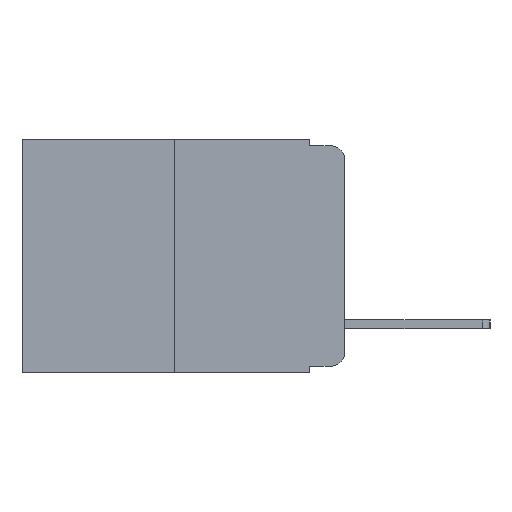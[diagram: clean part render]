
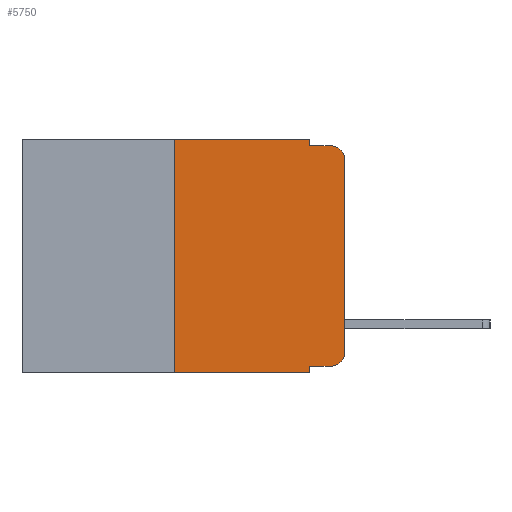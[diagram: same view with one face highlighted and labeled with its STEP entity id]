
A CAD part, left-side view. The second image highlights one B-rep face of the part: STEP entity #5750.
In plain terms, the highlighted planar face has unit normal (-1, 0, 0).
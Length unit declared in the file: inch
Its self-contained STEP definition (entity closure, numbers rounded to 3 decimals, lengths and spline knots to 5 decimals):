
#262 = DIRECTION ( 'NONE',  ( 0., -1., 0. ) ) ;
#375 = ORIENTED_EDGE ( 'NONE', *, *, #10968, .F. ) ;
#394 = ORIENTED_EDGE ( 'NONE', *, *, #12200, .T. ) ;
#423 = ORIENTED_EDGE ( 'NONE', *, *, #14077, .T. ) ;
#573 = DIRECTION ( 'NONE',  ( 0., 0., 1. ) ) ;
#577 = ORIENTED_EDGE ( 'NONE', *, *, #7756, .F. ) ;
#736 = LINE ( 'NONE', #17203, #4063 ) ;
#753 = VECTOR ( 'NONE', #2154, 39.37008 ) ;
#880 = FACE_OUTER_BOUND ( 'NONE', #13927, .T. ) ;
#1391 = CIRCLE ( 'NONE', #11927, 0.02 ) ;
#1457 = VECTOR ( 'NONE', #6926, 39.37008 ) ;
#1819 = EDGE_CURVE ( 'NONE', #5526, #11667, #8682, .T. ) ;
#2154 = DIRECTION ( 'NONE',  ( 0., -1., 0. ) ) ;
#2223 = DIRECTION ( 'NONE',  ( -1., 0., 0. ) ) ;
#2265 = CARTESIAN_POINT ( 'NONE',  ( 0., 0.051, -0.01 ) ) ;
#2388 = EDGE_CURVE ( 'NONE', #11225, #7381, #5765, .T. ) ;
#2497 = CARTESIAN_POINT ( 'NONE',  ( 0., 0.051, 0. ) ) ;
#2544 = ORIENTED_EDGE ( 'NONE', *, *, #2853, .T. ) ;
#2697 = DIRECTION ( 'NONE',  ( 1., 0., 0. ) ) ;
#2853 = EDGE_CURVE ( 'NONE', #13349, #5893, #15916, .T. ) ;
#2949 = CARTESIAN_POINT ( 'NONE',  ( 0., 0., -0.03 ) ) ;
#3145 = CARTESIAN_POINT ( 'NONE',  ( 0., 0.25, 0. ) ) ;
#3374 = VECTOR ( 'NONE', #5452, 39.37008 ) ;
#3471 = ORIENTED_EDGE ( 'NONE', *, *, #8211, .F. ) ;
#3778 = CARTESIAN_POINT ( 'NONE',  ( 0., 0.02, -0.03 ) ) ;
#4063 = VECTOR ( 'NONE', #573, 39.37008 ) ;
#4452 = EDGE_CURVE ( 'NONE', #11667, #6717, #1391, .T. ) ;
#4487 = CARTESIAN_POINT ( 'NONE',  ( 0., 0.051, -0.343 ) ) ;
#4535 = DIRECTION ( 'NONE',  ( -1., 0., 0. ) ) ;
#4559 = DIRECTION ( 'NONE',  ( 0., 0., -1. ) ) ;
#4885 = VECTOR ( 'NONE', #6963, 39.37008 ) ;
#4895 = VECTOR ( 'NONE', #16625, 39.37008 ) ;
#5059 = ORIENTED_EDGE ( 'NONE', *, *, #4452, .T. ) ;
#5452 = DIRECTION ( 'NONE',  ( 0., 0., -1. ) ) ;
#5526 = VERTEX_POINT ( 'NONE', #15768 ) ;
#5626 = CARTESIAN_POINT ( 'NONE',  ( 0., 0.02, -0.333 ) ) ;
#5638 = VECTOR ( 'NONE', #262, 39.37008 ) ;
#5750 = ADVANCED_FACE ( 'NONE', ( #880 ), #16596, .F. ) ;
#5765 = LINE ( 'NONE', #11553, #1457 ) ;
#5893 = VERTEX_POINT ( 'NONE', #4487 ) ;
#6717 = VERTEX_POINT ( 'NONE', #7292 ) ;
#6846 = CIRCLE ( 'NONE', #14888, 0.02 ) ;
#6926 = DIRECTION ( 'NONE',  ( 0., 0., -1. ) ) ;
#6963 = DIRECTION ( 'NONE',  ( 0., 0., 1. ) ) ;
#7292 = CARTESIAN_POINT ( 'NONE',  ( 0., 0.02, -0.01 ) ) ;
#7381 = VERTEX_POINT ( 'NONE', #2265 ) ;
#7756 = EDGE_CURVE ( 'NONE', #7381, #6717, #13536, .T. ) ;
#7896 = CARTESIAN_POINT ( 'NONE',  ( 0., 0., 0. ) ) ;
#7938 = LINE ( 'NONE', #10737, #753 ) ;
#7962 = ORIENTED_EDGE ( 'NONE', *, *, #1819, .T. ) ;
#8211 = EDGE_CURVE ( 'NONE', #11590, #5893, #14610, .T. ) ;
#8437 = VERTEX_POINT ( 'NONE', #3145 ) ;
#8682 = LINE ( 'NONE', #7896, #4885 ) ;
#9321 = ORIENTED_EDGE ( 'NONE', *, *, #11308, .F. ) ;
#10296 = CARTESIAN_POINT ( 'NONE',  ( 0., 0.051, 0. ) ) ;
#10561 = AXIS2_PLACEMENT_3D ( 'NONE', #11285, #2697, #12663 ) ;
#10737 = CARTESIAN_POINT ( 'NONE',  ( 0., 0.473, 0. ) ) ;
#10819 = CARTESIAN_POINT ( 'NONE',  ( 0., 0.02, -0.313 ) ) ;
#10968 = EDGE_CURVE ( 'NONE', #8437, #11225, #7938, .T. ) ;
#11091 = CARTESIAN_POINT ( 'NONE',  ( 0., 0.051, -0.333 ) ) ;
#11225 = VERTEX_POINT ( 'NONE', #10296 ) ;
#11285 = CARTESIAN_POINT ( 'NONE',  ( 0., 0.473, 0. ) ) ;
#11308 = EDGE_CURVE ( 'NONE', #13349, #8437, #736, .T. ) ;
#11553 = CARTESIAN_POINT ( 'NONE',  ( 0., 0.051, 0. ) ) ;
#11590 = VERTEX_POINT ( 'NONE', #11091 ) ;
#11648 = CARTESIAN_POINT ( 'NONE',  ( 0., 0.051, -0.01 ) ) ;
#11667 = VERTEX_POINT ( 'NONE', #2949 ) ;
#11927 = AXIS2_PLACEMENT_3D ( 'NONE', #3778, #4535, #4559 ) ;
#12200 = EDGE_CURVE ( 'NONE', #11590, #13752, #15533, .T. ) ;
#12211 = DIRECTION ( 'NONE',  ( 0., 0., -1. ) ) ;
#12663 = DIRECTION ( 'NONE',  ( 0., 0., -1. ) ) ;
#12774 = ORIENTED_EDGE ( 'NONE', *, *, #2388, .F. ) ;
#12777 = VECTOR ( 'NONE', #17599, 39.37008 ) ;
#13349 = VERTEX_POINT ( 'NONE', #17034 ) ;
#13536 = LINE ( 'NONE', #11648, #5638 ) ;
#13752 = VERTEX_POINT ( 'NONE', #5626 ) ;
#13927 = EDGE_LOOP ( 'NONE', ( #7962, #5059, #577, #12774, #375, #9321, #2544, #3471, #394, #423 ) ) ;
#14077 = EDGE_CURVE ( 'NONE', #13752, #5526, #6846, .T. ) ;
#14610 = LINE ( 'NONE', #2497, #3374 ) ;
#14888 = AXIS2_PLACEMENT_3D ( 'NONE', #10819, #2223, #12211 ) ;
#15332 = CARTESIAN_POINT ( 'NONE',  ( 0., 0.051, -0.333 ) ) ;
#15533 = LINE ( 'NONE', #15332, #4895 ) ;
#15768 = CARTESIAN_POINT ( 'NONE',  ( 0., 0., -0.313 ) ) ;
#15916 = LINE ( 'NONE', #17548, #12777 ) ;
#16596 = PLANE ( 'NONE',  #10561 ) ;
#16625 = DIRECTION ( 'NONE',  ( 0., -1., 0. ) ) ;
#17034 = CARTESIAN_POINT ( 'NONE',  ( 0., 0.25, -0.343 ) ) ;
#17203 = CARTESIAN_POINT ( 'NONE',  ( 0., 0.25, 0. ) ) ;
#17548 = CARTESIAN_POINT ( 'NONE',  ( 0., 0.473, -0.343 ) ) ;
#17599 = DIRECTION ( 'NONE',  ( 0., -1., 0. ) ) ;
